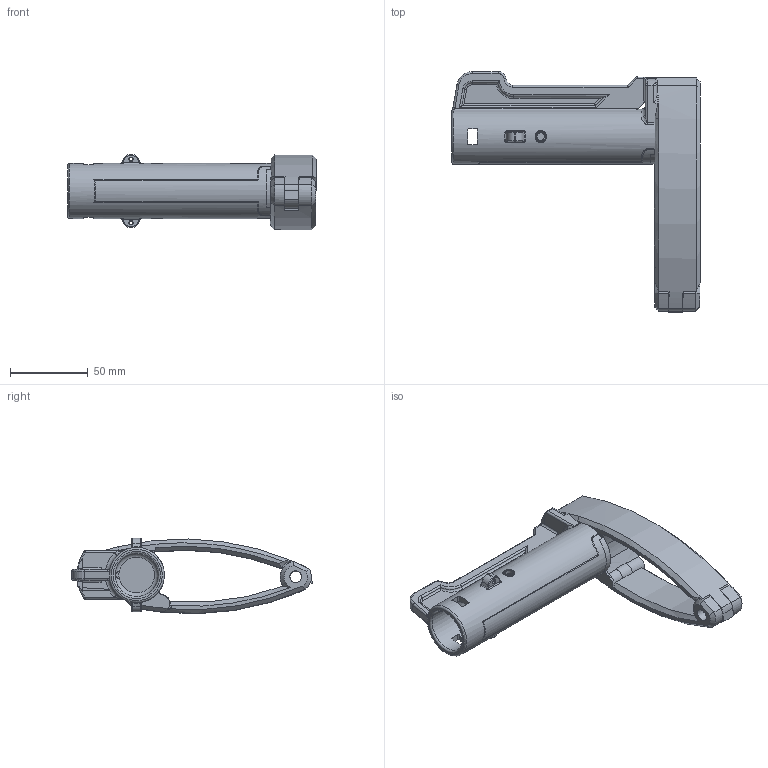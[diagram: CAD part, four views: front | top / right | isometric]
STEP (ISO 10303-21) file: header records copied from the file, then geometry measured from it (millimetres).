
FILE_DESCRIPTION(/* description */ (''),/* implementation_level */ '2;1');
FILE_NAME(/* name */ 'NotaStawk.step',/* time_stamp */ '2022-01-22T18:59:44-06:00',/* author */ (''),/* organization */ (''),/* preprocessor_version */ 'ST-DEVELOPER v18.1',/* originating_system */ 'Autodesk Translation Framework v10.13.0.1454',/* authorisation */ '');
FILE_SCHEMA (('AUTOMOTIVE_DESIGN { 1 0 10303 214 3 1 1 }'));
Length unit declared in the file: millimetre
Products named in the file (5): Stock V2; NotaStawk; Brace body;  Brace; Lever
Assembly tree (4 placements, depth 4):
  Stock V2
    NotaStawk
      Brace body
         Brace
        Lever
Bounding box: 159.65 x 154.81 x 48.54 mm (x, y, z)
Volume: 157977.8 mm3; surface area: 55078.9 mm2
Topology: 2 solids, 2 shells, 418 faces, 1094 edges, 691 vertices
Faces by surface type: plane 172, cylinder 128, bspline 58, torus 41, cone 19
Full cylindrical faces by diameter (mm): 2.286 x2, 4.826 x2, 7.65 x3, 27.813 x1, 35.433 x1
Entity records: 15183 total; most frequent: CARTESIAN_POINT 4992, ORIENTED_EDGE 2184, DIRECTION 2027, EDGE_CURVE 1092, AXIS2_PLACEMENT_3D 749, VERTEX_POINT 691, LINE 529, VECTOR 529
